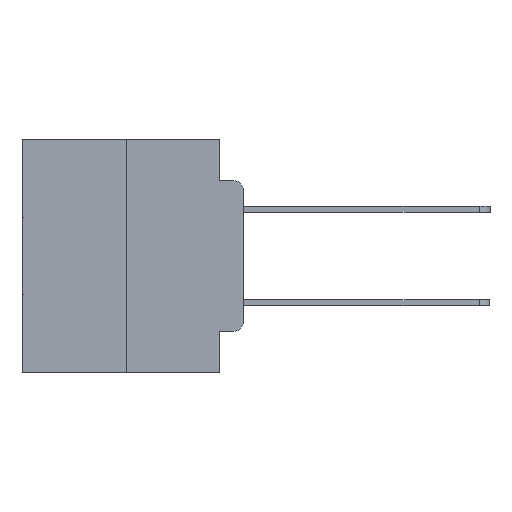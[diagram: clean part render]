
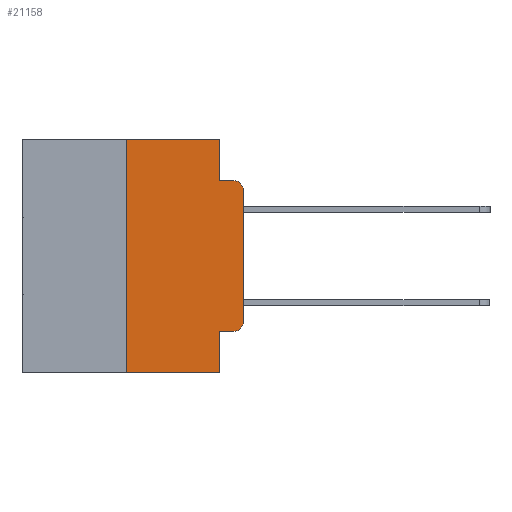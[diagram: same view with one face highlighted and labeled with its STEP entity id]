
A CAD part, left-side view. The second image highlights one B-rep face of the part: STEP entity #21158.
In plain terms, the highlighted planar face has unit normal (-1, 0, 0).
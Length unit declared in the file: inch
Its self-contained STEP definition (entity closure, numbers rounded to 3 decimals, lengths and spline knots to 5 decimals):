
#500 = CARTESIAN_POINT ( 'NONE',  ( 0., 0.02, -0.3915 ) ) ;
#645 = AXIS2_PLACEMENT_3D ( 'NONE', #1366, #12548, #27407 ) ;
#960 = ORIENTED_EDGE ( 'NONE', *, *, #11361, .T. ) ;
#991 = LINE ( 'NONE', #22465, #27121 ) ;
#1101 = LINE ( 'NONE', #8824, #27852 ) ;
#1366 = CARTESIAN_POINT ( 'NONE',  ( 0., 0.02, -0.1085 ) ) ;
#2047 = PLANE ( 'NONE',  #16267 ) ;
#2630 = CARTESIAN_POINT ( 'NONE',  ( 0., 0., 0. ) ) ;
#2706 = EDGE_LOOP ( 'NONE', ( #960, #13474, #25476, #10144, #17914, #21235, #10533, #22926, #7789, #14942 ) ) ;
#3151 = LINE ( 'NONE', #26488, #8406 ) ;
#3210 = CARTESIAN_POINT ( 'NONE',  ( 0., 0.02, -0.4115 ) ) ;
#3461 = VERTEX_POINT ( 'NONE', #3600 ) ;
#3600 = CARTESIAN_POINT ( 'NONE',  ( 0., 0.25, -0.5 ) ) ;
#3997 = CIRCLE ( 'NONE', #12239, 0.02 ) ;
#4317 = DIRECTION ( 'NONE',  ( 1., 0., 0. ) ) ;
#4766 = CARTESIAN_POINT ( 'NONE',  ( 0., 0., -0.3915 ) ) ;
#5110 = EDGE_CURVE ( 'NONE', #7750, #13889, #3997, .T. ) ;
#5481 = EDGE_CURVE ( 'NONE', #10339, #24150, #11892, .T. ) ;
#5674 = DIRECTION ( 'NONE',  ( -1., 0., 0. ) ) ;
#6048 = VECTOR ( 'NONE', #11834, 39.37008 ) ;
#6186 = LINE ( 'NONE', #9075, #11329 ) ;
#6236 = EDGE_CURVE ( 'NONE', #25199, #19142, #10160, .T. ) ;
#6815 = LINE ( 'NONE', #2630, #17683 ) ;
#6969 = EDGE_CURVE ( 'NONE', #27012, #24150, #3151, .T. ) ;
#7750 = VERTEX_POINT ( 'NONE', #3210 ) ;
#7789 = ORIENTED_EDGE ( 'NONE', *, *, #25812, .T. ) ;
#8406 = VECTOR ( 'NONE', #15836, 39.37008 ) ;
#8824 = CARTESIAN_POINT ( 'NONE',  ( 0., 0.051, -0.4115 ) ) ;
#9075 = CARTESIAN_POINT ( 'NONE',  ( 0., 0.051, 0. ) ) ;
#9671 = CARTESIAN_POINT ( 'NONE',  ( 0., 0.473, -0.5 ) ) ;
#9681 = DIRECTION ( 'NONE',  ( 0., 0., -1. ) ) ;
#10144 = ORIENTED_EDGE ( 'NONE', *, *, #20016, .F. ) ;
#10160 = LINE ( 'NONE', #24117, #20910 ) ;
#10339 = VERTEX_POINT ( 'NONE', #14422 ) ;
#10533 = ORIENTED_EDGE ( 'NONE', *, *, #26052, .T. ) ;
#11329 = VECTOR ( 'NONE', #19787, 39.37008 ) ;
#11361 = EDGE_CURVE ( 'NONE', #13889, #10339, #6815, .T. ) ;
#11477 = VERTEX_POINT ( 'NONE', #24680 ) ;
#11834 = DIRECTION ( 'NONE',  ( 0., -1., 0. ) ) ;
#11892 = CIRCLE ( 'NONE', #645, 0.02 ) ;
#12239 = AXIS2_PLACEMENT_3D ( 'NONE', #500, #5674, #9681 ) ;
#12548 = DIRECTION ( 'NONE',  ( -1., 0., 0. ) ) ;
#13361 = EDGE_CURVE ( 'NONE', #3461, #25199, #991, .T. ) ;
#13474 = ORIENTED_EDGE ( 'NONE', *, *, #5481, .T. ) ;
#13549 = CARTESIAN_POINT ( 'NONE',  ( 0., 0.02, -0.0885 ) ) ;
#13889 = VERTEX_POINT ( 'NONE', #4766 ) ;
#14422 = CARTESIAN_POINT ( 'NONE',  ( 0., 0., -0.1085 ) ) ;
#14507 = FACE_OUTER_BOUND ( 'NONE', #2706, .T. ) ;
#14772 = CARTESIAN_POINT ( 'NONE',  ( 0., 0.051, 0. ) ) ;
#14942 = ORIENTED_EDGE ( 'NONE', *, *, #5110, .T. ) ;
#15836 = DIRECTION ( 'NONE',  ( 0., -1., 0. ) ) ;
#16267 = AXIS2_PLACEMENT_3D ( 'NONE', #17396, #4317, #19523 ) ;
#16468 = CARTESIAN_POINT ( 'NONE',  ( 0., 0.051, 0. ) ) ;
#16737 = CARTESIAN_POINT ( 'NONE',  ( 0., 0.051, -0.0885 ) ) ;
#17396 = CARTESIAN_POINT ( 'NONE',  ( 0., 0.473, 0. ) ) ;
#17683 = VECTOR ( 'NONE', #20078, 39.37008 ) ;
#17699 = EDGE_CURVE ( 'NONE', #11477, #27233, #26155, .T. ) ;
#17914 = ORIENTED_EDGE ( 'NONE', *, *, #6236, .F. ) ;
#18592 = DIRECTION ( 'NONE',  ( 0., 0., -1. ) ) ;
#19142 = VERTEX_POINT ( 'NONE', #14772 ) ;
#19523 = DIRECTION ( 'NONE',  ( 0., 0., -1. ) ) ;
#19546 = DIRECTION ( 'NONE',  ( 0., -1., 0. ) ) ;
#19787 = DIRECTION ( 'NONE',  ( 0., 0., -1. ) ) ;
#20016 = EDGE_CURVE ( 'NONE', #19142, #27012, #6186, .T. ) ;
#20078 = DIRECTION ( 'NONE',  ( 0., 0., 1. ) ) ;
#20910 = VECTOR ( 'NONE', #26255, 39.37008 ) ;
#21158 = ADVANCED_FACE ( 'NONE', ( #14507 ), #2047, .F. ) ;
#21235 = ORIENTED_EDGE ( 'NONE', *, *, #13361, .F. ) ;
#21744 = CARTESIAN_POINT ( 'NONE',  ( 0., 0.051, -0.5 ) ) ;
#22465 = CARTESIAN_POINT ( 'NONE',  ( 0., 0.25, 0. ) ) ;
#22926 = ORIENTED_EDGE ( 'NONE', *, *, #17699, .F. ) ;
#23245 = LINE ( 'NONE', #9671, #6048 ) ;
#24117 = CARTESIAN_POINT ( 'NONE',  ( 0., 0.473, 0. ) ) ;
#24150 = VERTEX_POINT ( 'NONE', #13549 ) ;
#24573 = DIRECTION ( 'NONE',  ( 0., 0., 1. ) ) ;
#24680 = CARTESIAN_POINT ( 'NONE',  ( 0., 0.051, -0.4115 ) ) ;
#25199 = VERTEX_POINT ( 'NONE', #27950 ) ;
#25475 = VECTOR ( 'NONE', #18592, 39.37008 ) ;
#25476 = ORIENTED_EDGE ( 'NONE', *, *, #6969, .F. ) ;
#25812 = EDGE_CURVE ( 'NONE', #11477, #7750, #1101, .T. ) ;
#26052 = EDGE_CURVE ( 'NONE', #3461, #27233, #23245, .T. ) ;
#26155 = LINE ( 'NONE', #16468, #25475 ) ;
#26255 = DIRECTION ( 'NONE',  ( 0., -1., 0. ) ) ;
#26488 = CARTESIAN_POINT ( 'NONE',  ( 0., 0.051, -0.0885 ) ) ;
#27012 = VERTEX_POINT ( 'NONE', #16737 ) ;
#27121 = VECTOR ( 'NONE', #24573, 39.37008 ) ;
#27233 = VERTEX_POINT ( 'NONE', #21744 ) ;
#27407 = DIRECTION ( 'NONE',  ( 0., 0., -1. ) ) ;
#27852 = VECTOR ( 'NONE', #19546, 39.37008 ) ;
#27950 = CARTESIAN_POINT ( 'NONE',  ( 0., 0.25, 0. ) ) ;
